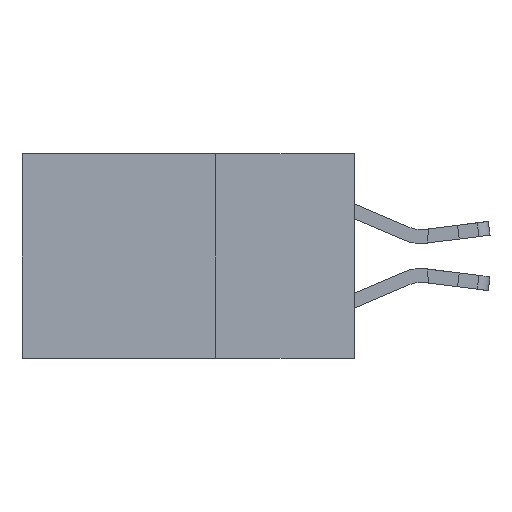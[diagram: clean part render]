
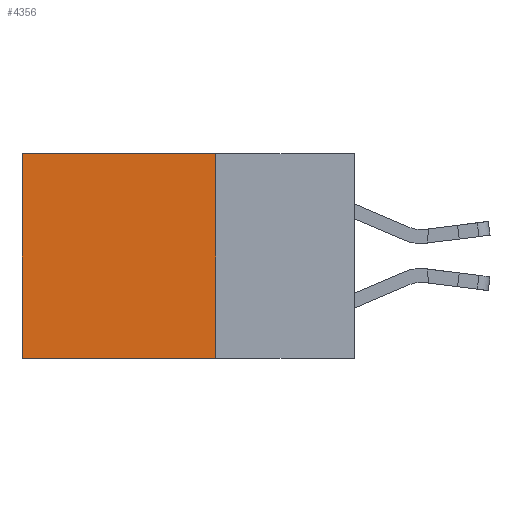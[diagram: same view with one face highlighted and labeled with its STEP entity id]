
A CAD part, left-side view. The second image highlights one B-rep face of the part: STEP entity #4356.
In plain terms, the highlighted planar face has unit normal (-1, 0, 0).
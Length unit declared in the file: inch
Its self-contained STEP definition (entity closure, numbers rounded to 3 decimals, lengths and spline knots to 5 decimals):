
#119 = ORIENTED_EDGE ( 'NONE', *, *, #1802, .T. ) ;
#167 = VERTEX_POINT ( 'NONE', #4291 ) ;
#386 = EDGE_LOOP ( 'NONE', ( #119, #5861, #7228, #11937 ) ) ;
#476 = CARTESIAN_POINT ( 'NONE',  ( 0.2615, 0.6, 0. ) ) ;
#914 = CARTESIAN_POINT ( 'NONE',  ( 0.2615, 0.6, -0.37 ) ) ;
#1030 = VERTEX_POINT ( 'NONE', #476 ) ;
#1113 = EDGE_CURVE ( 'NONE', #1366, #1030, #6589, .T. ) ;
#1298 = DIRECTION ( 'NONE',  ( 0., 0., -1. ) ) ;
#1366 = VERTEX_POINT ( 'NONE', #4916 ) ;
#1487 = EDGE_CURVE ( 'NONE', #7783, #167, #7496, .T. ) ;
#1802 = EDGE_CURVE ( 'NONE', #1030, #167, #6959, .T. ) ;
#2219 = PLANE ( 'NONE',  #11418 ) ;
#4291 = CARTESIAN_POINT ( 'NONE',  ( 0.2615, 0.6, -0.37 ) ) ;
#4356 = ADVANCED_FACE ( 'NONE', ( #11228 ), #2219, .F. ) ;
#4916 = CARTESIAN_POINT ( 'NONE',  ( 0.2615, 0.25, 0. ) ) ;
#5444 = CARTESIAN_POINT ( 'NONE',  ( 0.2615, 0.25, -0.37 ) ) ;
#5512 = CARTESIAN_POINT ( 'NONE',  ( 0.2615, 0.25, 0. ) ) ;
#5861 = ORIENTED_EDGE ( 'NONE', *, *, #1487, .F. ) ;
#5974 = CARTESIAN_POINT ( 'NONE',  ( 0.2615, 0.25, -0.37 ) ) ;
#6246 = CARTESIAN_POINT ( 'NONE',  ( 0.2615, 0.25, -0.37 ) ) ;
#6331 = DIRECTION ( 'NONE',  ( 0., 1., 0. ) ) ;
#6589 = LINE ( 'NONE', #5512, #12560 ) ;
#6676 = VECTOR ( 'NONE', #7884, 39.37008 ) ;
#6959 = LINE ( 'NONE', #914, #6676 ) ;
#7228 = ORIENTED_EDGE ( 'NONE', *, *, #10741, .F. ) ;
#7496 = LINE ( 'NONE', #12365, #10127 ) ;
#7783 = VERTEX_POINT ( 'NONE', #5974 ) ;
#7884 = DIRECTION ( 'NONE',  ( 0., 0., -1. ) ) ;
#8363 = LINE ( 'NONE', #5444, #10240 ) ;
#8470 = DIRECTION ( 'NONE',  ( 0., 1., 0. ) ) ;
#10127 = VECTOR ( 'NONE', #8470, 39.37008 ) ;
#10240 = VECTOR ( 'NONE', #12383, 39.37008 ) ;
#10315 = DIRECTION ( 'NONE',  ( 1., 0., 0. ) ) ;
#10741 = EDGE_CURVE ( 'NONE', #1366, #7783, #8363, .T. ) ;
#11228 = FACE_OUTER_BOUND ( 'NONE', #386, .T. ) ;
#11418 = AXIS2_PLACEMENT_3D ( 'NONE', #6246, #10315, #1298 ) ;
#11937 = ORIENTED_EDGE ( 'NONE', *, *, #1113, .T. ) ;
#12365 = CARTESIAN_POINT ( 'NONE',  ( 0.2615, 0.25, -0.37 ) ) ;
#12383 = DIRECTION ( 'NONE',  ( 0., 0., -1. ) ) ;
#12560 = VECTOR ( 'NONE', #6331, 39.37008 ) ;
